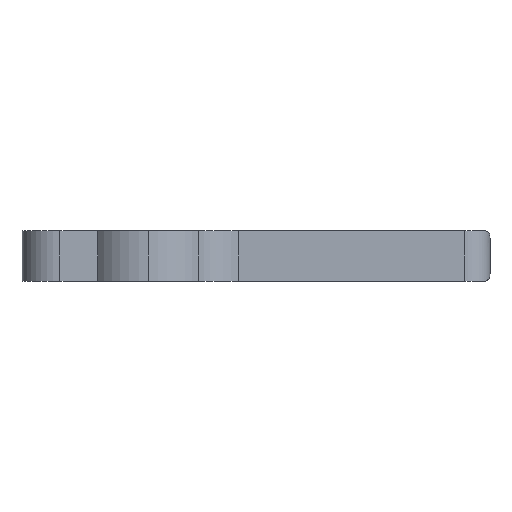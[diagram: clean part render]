
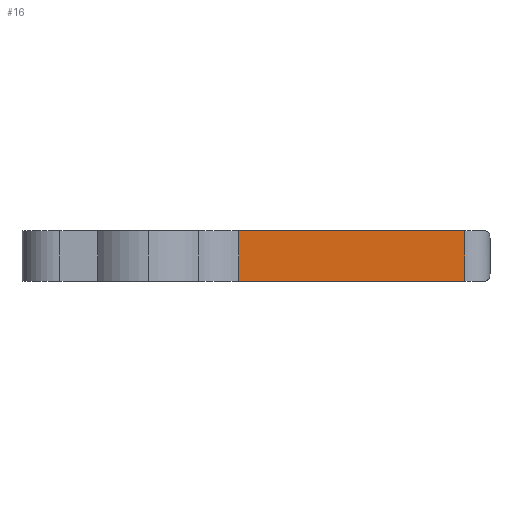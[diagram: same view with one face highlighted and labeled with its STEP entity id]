
A CAD part, left-side view. The second image highlights one B-rep face of the part: STEP entity #16.
In plain terms, the highlighted planar face has unit normal (-1, 0, 0).
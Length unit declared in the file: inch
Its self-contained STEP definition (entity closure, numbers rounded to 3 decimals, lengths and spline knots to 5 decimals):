
#16 = ADVANCED_FACE ( 'NONE', ( #965 ), #1167, .F. ) ;
#34 = VERTEX_POINT ( 'NONE', #1212 ) ;
#248 = DIRECTION ( 'NONE',  ( 0., 0., -1. ) ) ;
#280 = DIRECTION ( 'NONE',  ( 0., 1., 0. ) ) ;
#337 = CARTESIAN_POINT ( 'NONE',  ( -0.075, 0., 0. ) ) ;
#355 = LINE ( 'NONE', #1004, #1294 ) ;
#401 = CARTESIAN_POINT ( 'NONE',  ( -0.075, -1.45, 0. ) ) ;
#423 = EDGE_CURVE ( 'NONE', #1278, #1050, #432, .T. ) ;
#432 = LINE ( 'NONE', #1112, #1253 ) ;
#456 = VECTOR ( 'NONE', #248, 39.37008 ) ;
#487 = DIRECTION ( 'NONE',  ( 1., 0., 0. ) ) ;
#635 = EDGE_CURVE ( 'NONE', #1533, #34, #355, .T. ) ;
#817 = ORIENTED_EDGE ( 'NONE', *, *, #1656, .T. ) ;
#828 = CARTESIAN_POINT ( 'NONE',  ( -0.075, -1.45, 0.2 ) ) ;
#879 = ORIENTED_EDGE ( 'NONE', *, *, #635, .F. ) ;
#965 = FACE_OUTER_BOUND ( 'NONE', #1453, .T. ) ;
#968 = EDGE_CURVE ( 'NONE', #1050, #34, #1160, .T. ) ;
#1004 = CARTESIAN_POINT ( 'NONE',  ( -0.075, 0., 0. ) ) ;
#1050 = VERTEX_POINT ( 'NONE', #1110 ) ;
#1053 = ORIENTED_EDGE ( 'NONE', *, *, #423, .T. ) ;
#1110 = CARTESIAN_POINT ( 'NONE',  ( -0.075, -0.5562, 0.2 ) ) ;
#1112 = CARTESIAN_POINT ( 'NONE',  ( -0.075, 0., 0.2 ) ) ;
#1116 = VECTOR ( 'NONE', #1655, 39.37008 ) ;
#1158 = AXIS2_PLACEMENT_3D ( 'NONE', #337, #487, #1446 ) ;
#1160 = LINE ( 'NONE', #1769, #456 ) ;
#1167 = PLANE ( 'NONE',  #1158 ) ;
#1212 = CARTESIAN_POINT ( 'NONE',  ( -0.075, -0.5562, 0. ) ) ;
#1253 = VECTOR ( 'NONE', #280, 39.37008 ) ;
#1278 = VERTEX_POINT ( 'NONE', #1707 ) ;
#1294 = VECTOR ( 'NONE', #1568, 39.37008 ) ;
#1446 = DIRECTION ( 'NONE',  ( 0., 0., -1. ) ) ;
#1453 = EDGE_LOOP ( 'NONE', ( #879, #817, #1053, #1663 ) ) ;
#1533 = VERTEX_POINT ( 'NONE', #401 ) ;
#1568 = DIRECTION ( 'NONE',  ( 0., 1., 0. ) ) ;
#1569 = LINE ( 'NONE', #828, #1116 ) ;
#1655 = DIRECTION ( 'NONE',  ( 0., 0., 1. ) ) ;
#1656 = EDGE_CURVE ( 'NONE', #1533, #1278, #1569, .T. ) ;
#1663 = ORIENTED_EDGE ( 'NONE', *, *, #968, .T. ) ;
#1707 = CARTESIAN_POINT ( 'NONE',  ( -0.075, -1.45, 0.2 ) ) ;
#1769 = CARTESIAN_POINT ( 'NONE',  ( -0.075, -0.5562, 0. ) ) ;
